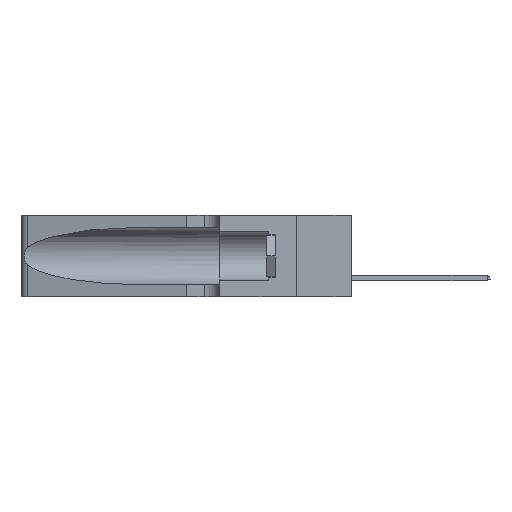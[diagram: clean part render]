
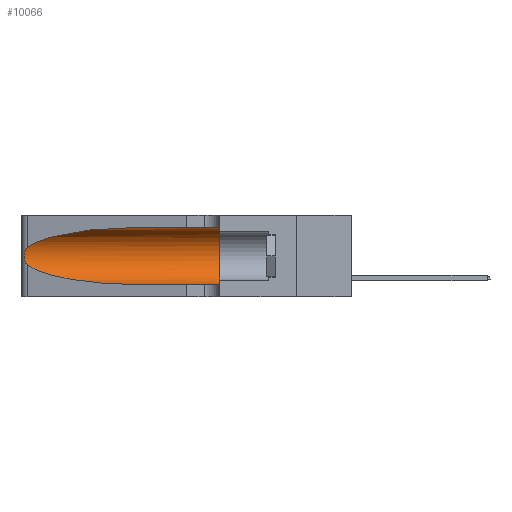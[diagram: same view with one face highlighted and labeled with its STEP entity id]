
A CAD part, left-side view. The second image highlights one B-rep face of the part: STEP entity #10066.
In plain terms, the highlighted cylindrical face has radius 3.308 mm (diameter 6.617 mm), a partial arc.
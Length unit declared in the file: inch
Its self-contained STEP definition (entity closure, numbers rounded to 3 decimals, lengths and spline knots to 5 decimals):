
#15 =( BOUNDED_CURVE ( )  B_SPLINE_CURVE ( 3, ( #32059, #22193, #18742, #14275 ),
 .UNSPECIFIED., .F., .F. ) 
 B_SPLINE_CURVE_WITH_KNOTS ( ( 4, 4 ),
 ( 3.44316, 4.71239 ),
 .UNSPECIFIED. ) 
 CURVE ( )  GEOMETRIC_REPRESENTATION_ITEM ( )  RATIONAL_B_SPLINE_CURVE ( ( 1., 0.87, 0.87, 1. ) ) 
 REPRESENTATION_ITEM ( '' )  );
#138 = VERTEX_POINT ( 'NONE', #22908 ) ;
#647 = CARTESIAN_POINT ( 'NONE',  ( 0.25789, 1.23486, 0.15765 ) ) ;
#2169 = ORIENTED_EDGE ( 'NONE', *, *, #15337, .F. ) ;
#2386 = CARTESIAN_POINT ( 'NONE',  ( 0.1305, 0.72297, 0.31525 ) ) ;
#3089 = ORIENTED_EDGE ( 'NONE', *, *, #16118, .T. ) ;
#3110 = DIRECTION ( 'NONE',  ( 0., 0., -1. ) ) ;
#4589 = EDGE_CURVE ( 'NONE', #32099, #30299, #7340, .T. ) ;
#6688 = DIRECTION ( 'NONE',  ( 0., -1., 0. ) ) ;
#7330 = CARTESIAN_POINT ( 'NONE',  ( 0.25487, 1.22718, 0.22369 ) ) ;
#7340 =( BOUNDED_CURVE ( )  B_SPLINE_CURVE ( 3, ( #2386, #19383, #29129, #39322 ),
 .UNSPECIFIED., .F., .T. ) 
 B_SPLINE_CURVE_WITH_KNOTS ( ( 4, 4 ),
 ( 1.5708, 2.84003 ),
 .UNSPECIFIED. ) 
 CURVE ( )  GEOMETRIC_REPRESENTATION_ITEM ( )  RATIONAL_B_SPLINE_CURVE ( ( 1., 0.87, 0.87, 1. ) ) 
 REPRESENTATION_ITEM ( '' )  );
#7774 = CARTESIAN_POINT ( 'NONE',  ( 0.26075, 1.23896, 0.178 ) ) ;
#9244 = FACE_OUTER_BOUND ( 'NONE', #13464, .T. ) ;
#9263 = B_SPLINE_CURVE_WITH_KNOTS ( 'NONE', 3,
 ( #7330, #27834, #24389, #17332, #14352, #34705, #28130, #7774, #31249, #27972, #647, #14212, #38025, #24529 ),
 .UNSPECIFIED., .F., .F.,
 ( 4, 2, 2, 2, 2, 2, 4 ),
 ( 0., 0.00027, 0.00053, 0.00107, 0.0016, 0.00187, 0.00214 ),
 .UNSPECIFIED. ) ;
#10066 = ADVANCED_FACE ( 'NONE', ( #9244 ), #11888, .F. ) ;
#10288 = VERTEX_POINT ( 'NONE', #24022 ) ;
#10470 = VERTEX_POINT ( 'NONE', #12624 ) ;
#10489 = VECTOR ( 'NONE', #12721, 39.37008 ) ;
#11329 = ORIENTED_EDGE ( 'NONE', *, *, #39103, .T. ) ;
#11888 = CYLINDRICAL_SURFACE ( 'NONE', #38773, 0.13025 ) ;
#12624 = CARTESIAN_POINT ( 'NONE',  ( 0.1305, 0.35, 0.31525 ) ) ;
#12721 = DIRECTION ( 'NONE',  ( 0., -1., 0. ) ) ;
#13464 = EDGE_LOOP ( 'NONE', ( #40205, #40896, #11329, #3089, #2169, #22309 ) ) ;
#13497 = CARTESIAN_POINT ( 'NONE',  ( 0.25487, 1.22718, 0.14631 ) ) ;
#14212 = CARTESIAN_POINT ( 'NONE',  ( 0.25639, 1.23186, 0.15144 ) ) ;
#14275 = CARTESIAN_POINT ( 'NONE',  ( 0.1305, 0.72297, 0.05475 ) ) ;
#14352 = CARTESIAN_POINT ( 'NONE',  ( 0.25854, 1.2359, 0.20912 ) ) ;
#14869 = CIRCLE ( 'NONE', #40214, 0.13025 ) ;
#15337 = EDGE_CURVE ( 'NONE', #10470, #10288, #14869, .T. ) ;
#15868 = VERTEX_POINT ( 'NONE', #13497 ) ;
#16118 = EDGE_CURVE ( 'NONE', #138, #10288, #32991, .T. ) ;
#17332 = CARTESIAN_POINT ( 'NONE',  ( 0.25787, 1.23484, 0.2124 ) ) ;
#17429 = DIRECTION ( 'NONE',  ( 0., 0., 1. ) ) ;
#18742 = CARTESIAN_POINT ( 'NONE',  ( 0.18966, 0.96281, 0.05475 ) ) ;
#19383 = CARTESIAN_POINT ( 'NONE',  ( 0.18966, 0.96281, 0.31525 ) ) ;
#20714 = DIRECTION ( 'NONE',  ( 0., 1., 0. ) ) ;
#22193 = CARTESIAN_POINT ( 'NONE',  ( 0.2373, 1.15595, 0.08982 ) ) ;
#22309 = ORIENTED_EDGE ( 'NONE', *, *, #22572, .F. ) ;
#22572 = EDGE_CURVE ( 'NONE', #32099, #10470, #25466, .T. ) ;
#22908 = CARTESIAN_POINT ( 'NONE',  ( 0.1305, 0.72297, 0.05475 ) ) ;
#24022 = CARTESIAN_POINT ( 'NONE',  ( 0.1305, 0.35, 0.05475 ) ) ;
#24389 = CARTESIAN_POINT ( 'NONE',  ( 0.25639, 1.23184, 0.21858 ) ) ;
#24529 = CARTESIAN_POINT ( 'NONE',  ( 0.25487, 1.22718, 0.14631 ) ) ;
#25466 = LINE ( 'NONE', #36829, #10489 ) ;
#26274 = DIRECTION ( 'NONE',  ( 0., -1., 0. ) ) ;
#27500 = CARTESIAN_POINT ( 'NONE',  ( 0.1305, 1.61858, 0.05475 ) ) ;
#27834 = CARTESIAN_POINT ( 'NONE',  ( 0.25555, 1.22994, 0.2215 ) ) ;
#27838 = CARTESIAN_POINT ( 'NONE',  ( 0.1305, 0.72297, 0.31525 ) ) ;
#27972 = CARTESIAN_POINT ( 'NONE',  ( 0.25856, 1.23593, 0.16098 ) ) ;
#28130 = CARTESIAN_POINT ( 'NONE',  ( 0.26075, 1.23896, 0.19203 ) ) ;
#28172 = EDGE_CURVE ( 'NONE', #30299, #15868, #9263, .T. ) ;
#29129 = CARTESIAN_POINT ( 'NONE',  ( 0.2373, 1.15595, 0.28018 ) ) ;
#30299 = VERTEX_POINT ( 'NONE', #43402 ) ;
#31249 = CARTESIAN_POINT ( 'NONE',  ( 0.26017, 1.23833, 0.17102 ) ) ;
#31903 = VECTOR ( 'NONE', #26274, 39.37008 ) ;
#32059 = CARTESIAN_POINT ( 'NONE',  ( 0.25487, 1.22718, 0.14631 ) ) ;
#32099 = VERTEX_POINT ( 'NONE', #27838 ) ;
#32991 = LINE ( 'NONE', #27500, #31903 ) ;
#34705 = CARTESIAN_POINT ( 'NONE',  ( 0.26018, 1.23835, 0.19895 ) ) ;
#36829 = CARTESIAN_POINT ( 'NONE',  ( 0.1305, 1.61858, 0.31525 ) ) ;
#38025 = CARTESIAN_POINT ( 'NONE',  ( 0.25555, 1.22993, 0.14849 ) ) ;
#38256 = CARTESIAN_POINT ( 'NONE',  ( 0.1305, 0.35, 0.185 ) ) ;
#38773 = AXIS2_PLACEMENT_3D ( 'NONE', #44247, #6688, #3110 ) ;
#39103 = EDGE_CURVE ( 'NONE', #15868, #138, #15, .T. ) ;
#39322 = CARTESIAN_POINT ( 'NONE',  ( 0.25487, 1.22718, 0.22369 ) ) ;
#40205 = ORIENTED_EDGE ( 'NONE', *, *, #4589, .T. ) ;
#40214 = AXIS2_PLACEMENT_3D ( 'NONE', #38256, #20714, #17429 ) ;
#40896 = ORIENTED_EDGE ( 'NONE', *, *, #28172, .T. ) ;
#43402 = CARTESIAN_POINT ( 'NONE',  ( 0.25487, 1.22718, 0.22369 ) ) ;
#44247 = CARTESIAN_POINT ( 'NONE',  ( 0.1305, 1.61858, 0.185 ) ) ;
